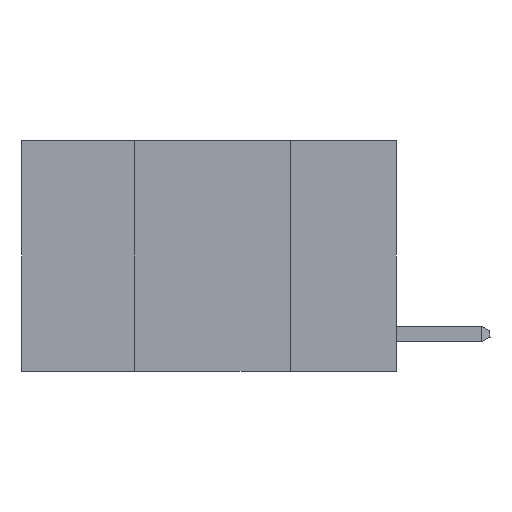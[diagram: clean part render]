
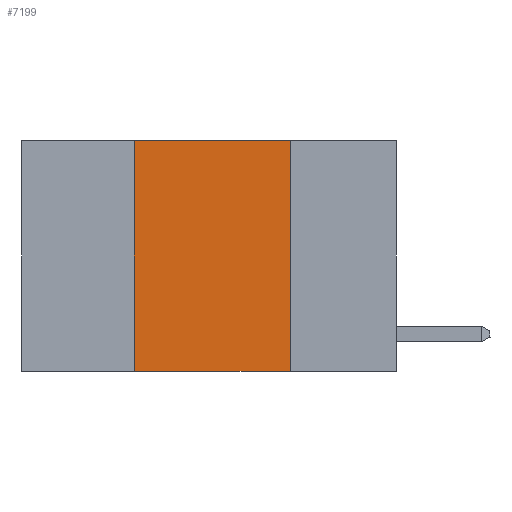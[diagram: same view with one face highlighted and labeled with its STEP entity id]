
A CAD part, left-side view. The second image highlights one B-rep face of the part: STEP entity #7199.
In plain terms, the highlighted planar face has unit normal (-1, 0, 0).
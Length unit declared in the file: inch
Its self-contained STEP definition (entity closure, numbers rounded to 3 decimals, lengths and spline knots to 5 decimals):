
#102 = CARTESIAN_POINT ( 'NONE',  ( 0., 0.42, 0. ) ) ;
#332 = EDGE_CURVE ( 'NONE', #12433, #16765, #18933, .T. ) ;
#1182 = CARTESIAN_POINT ( 'NONE',  ( 0., 0.6, 0. ) ) ;
#1300 = VECTOR ( 'NONE', #14799, 39.37008 ) ;
#1713 = LINE ( 'NONE', #9454, #12280 ) ;
#1850 = DIRECTION ( 'NONE',  ( 0., -1., 0. ) ) ;
#5182 = DIRECTION ( 'NONE',  ( 0., 0., -1. ) ) ;
#5304 = FACE_OUTER_BOUND ( 'NONE', #10407, .T. ) ;
#6662 = VERTEX_POINT ( 'NONE', #24136 ) ;
#6783 = VERTEX_POINT ( 'NONE', #7599 ) ;
#7199 = ADVANCED_FACE ( 'NONE', ( #5304 ), #10848, .F. ) ;
#7330 = CARTESIAN_POINT ( 'NONE',  ( 0., 0.17, 0. ) ) ;
#7493 = ORIENTED_EDGE ( 'NONE', *, *, #15991, .F. ) ;
#7599 = CARTESIAN_POINT ( 'NONE',  ( 0., 0.42, -0.37 ) ) ;
#7903 = CARTESIAN_POINT ( 'NONE',  ( 0., 0.17, -0.37 ) ) ;
#8130 = LINE ( 'NONE', #102, #11303 ) ;
#8429 = CARTESIAN_POINT ( 'NONE',  ( 0., 0.17, 0. ) ) ;
#9454 = CARTESIAN_POINT ( 'NONE',  ( 0., 0.6, -0.37 ) ) ;
#9733 = EDGE_CURVE ( 'NONE', #6783, #16765, #1713, .T. ) ;
#9790 = DIRECTION ( 'NONE',  ( 0., 0., 1. ) ) ;
#10407 = EDGE_LOOP ( 'NONE', ( #10898, #13795, #7493, #21732 ) ) ;
#10848 = PLANE ( 'NONE',  #18240 ) ;
#10898 = ORIENTED_EDGE ( 'NONE', *, *, #332, .F. ) ;
#11088 = DIRECTION ( 'NONE',  ( 0., -1., 0. ) ) ;
#11303 = VECTOR ( 'NONE', #9790, 39.37008 ) ;
#12280 = VECTOR ( 'NONE', #1850, 39.37008 ) ;
#12433 = VERTEX_POINT ( 'NONE', #8429 ) ;
#12907 = LINE ( 'NONE', #22953, #15822 ) ;
#13184 = DIRECTION ( 'NONE',  ( 1., 0., 0. ) ) ;
#13795 = ORIENTED_EDGE ( 'NONE', *, *, #25055, .F. ) ;
#14799 = DIRECTION ( 'NONE',  ( 0., 0., -1. ) ) ;
#15822 = VECTOR ( 'NONE', #11088, 39.37008 ) ;
#15991 = EDGE_CURVE ( 'NONE', #6783, #6662, #8130, .T. ) ;
#16765 = VERTEX_POINT ( 'NONE', #7903 ) ;
#18240 = AXIS2_PLACEMENT_3D ( 'NONE', #1182, #13184, #5182 ) ;
#18933 = LINE ( 'NONE', #7330, #1300 ) ;
#21732 = ORIENTED_EDGE ( 'NONE', *, *, #9733, .T. ) ;
#22953 = CARTESIAN_POINT ( 'NONE',  ( 0., 0.6, 0. ) ) ;
#24136 = CARTESIAN_POINT ( 'NONE',  ( 0., 0.42, 0. ) ) ;
#25055 = EDGE_CURVE ( 'NONE', #6662, #12433, #12907, .T. ) ;
